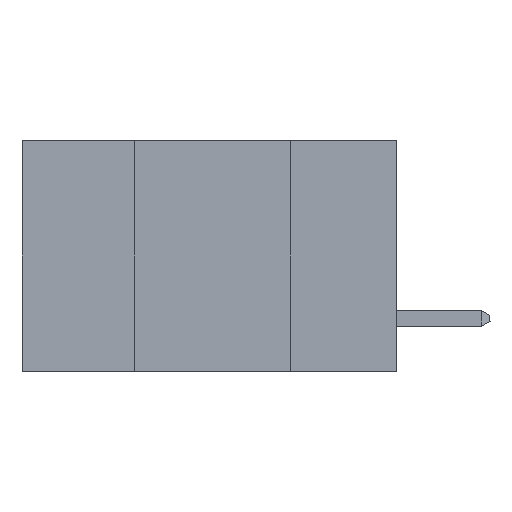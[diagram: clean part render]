
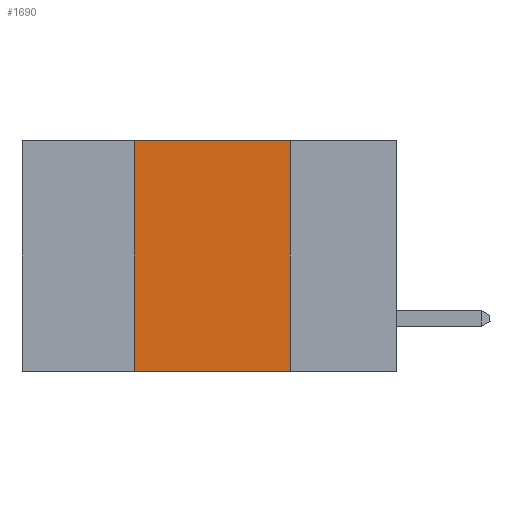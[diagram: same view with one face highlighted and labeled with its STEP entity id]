
A CAD part, left-side view. The second image highlights one B-rep face of the part: STEP entity #1690.
In plain terms, the highlighted planar face has unit normal (-1, 0, 0).
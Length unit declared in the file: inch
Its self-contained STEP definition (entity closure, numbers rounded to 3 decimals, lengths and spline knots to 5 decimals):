
#449 = LINE ( 'NONE', #28139, #11431 ) ;
#1614 = EDGE_CURVE ( 'NONE', #27212, #7978, #13308, .T. ) ;
#1690 = ADVANCED_FACE ( 'NONE', ( #4710 ), #5192, .F. ) ;
#1802 = CARTESIAN_POINT ( 'NONE',  ( 0., 0.6, 0. ) ) ;
#2137 = VECTOR ( 'NONE', #21023, 39.37008 ) ;
#2173 = DIRECTION ( 'NONE',  ( 1., 0., 0. ) ) ;
#2974 = CARTESIAN_POINT ( 'NONE',  ( 0., 0.17, 0. ) ) ;
#3393 = DIRECTION ( 'NONE',  ( 0., 0., -1. ) ) ;
#3789 = EDGE_CURVE ( 'NONE', #13405, #27212, #449, .T. ) ;
#4710 = FACE_OUTER_BOUND ( 'NONE', #23972, .T. ) ;
#5192 = PLANE ( 'NONE',  #13050 ) ;
#6419 = ORIENTED_EDGE ( 'NONE', *, *, #1614, .F. ) ;
#7547 = VECTOR ( 'NONE', #17100, 39.37008 ) ;
#7978 = VERTEX_POINT ( 'NONE', #27881 ) ;
#11431 = VECTOR ( 'NONE', #28045, 39.37008 ) ;
#11528 = EDGE_CURVE ( 'NONE', #12549, #13405, #19814, .T. ) ;
#12549 = VERTEX_POINT ( 'NONE', #18272 ) ;
#13050 = AXIS2_PLACEMENT_3D ( 'NONE', #1802, #2173, #3393 ) ;
#13308 = LINE ( 'NONE', #17010, #24282 ) ;
#13405 = VERTEX_POINT ( 'NONE', #23347 ) ;
#13587 = ORIENTED_EDGE ( 'NONE', *, *, #11528, .F. ) ;
#14470 = LINE ( 'NONE', #14643, #2137 ) ;
#14643 = CARTESIAN_POINT ( 'NONE',  ( 0., 0.6, -0.37 ) ) ;
#15978 = ORIENTED_EDGE ( 'NONE', *, *, #3789, .F. ) ;
#16942 = CARTESIAN_POINT ( 'NONE',  ( 0., 0.42, 0. ) ) ;
#17010 = CARTESIAN_POINT ( 'NONE',  ( 0., 0.17, 0. ) ) ;
#17100 = DIRECTION ( 'NONE',  ( 0., 0., 1. ) ) ;
#17775 = DIRECTION ( 'NONE',  ( 0., 0., -1. ) ) ;
#18272 = CARTESIAN_POINT ( 'NONE',  ( 0., 0.42, -0.37 ) ) ;
#19343 = EDGE_CURVE ( 'NONE', #12549, #7978, #14470, .T. ) ;
#19814 = LINE ( 'NONE', #16942, #7547 ) ;
#21023 = DIRECTION ( 'NONE',  ( 0., -1., 0. ) ) ;
#23201 = ORIENTED_EDGE ( 'NONE', *, *, #19343, .T. ) ;
#23347 = CARTESIAN_POINT ( 'NONE',  ( 0., 0.42, 0. ) ) ;
#23972 = EDGE_LOOP ( 'NONE', ( #6419, #15978, #13587, #23201 ) ) ;
#24282 = VECTOR ( 'NONE', #17775, 39.37008 ) ;
#27212 = VERTEX_POINT ( 'NONE', #2974 ) ;
#27881 = CARTESIAN_POINT ( 'NONE',  ( 0., 0.17, -0.37 ) ) ;
#28045 = DIRECTION ( 'NONE',  ( 0., -1., 0. ) ) ;
#28139 = CARTESIAN_POINT ( 'NONE',  ( 0., 0.6, 0. ) ) ;
